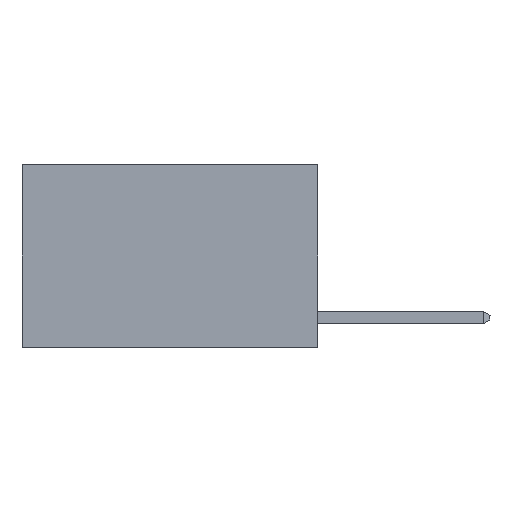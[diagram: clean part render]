
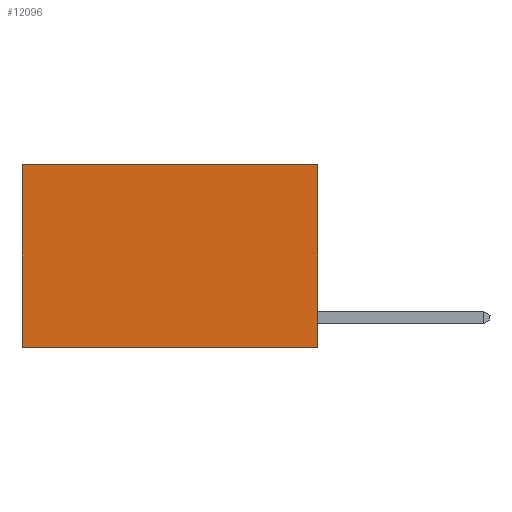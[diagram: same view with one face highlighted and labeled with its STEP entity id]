
A CAD part, left-side view. The second image highlights one B-rep face of the part: STEP entity #12096.
In plain terms, the highlighted planar face has unit normal (-1, 0, 0).
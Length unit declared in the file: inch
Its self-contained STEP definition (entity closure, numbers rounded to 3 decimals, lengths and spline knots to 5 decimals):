
#21 = LINE ( 'NONE', #401, #19808 ) ;
#174 = FACE_OUTER_BOUND ( 'NONE', #12239, .T. ) ;
#401 = CARTESIAN_POINT ( 'NONE',  ( 0.2625, 0., 0. ) ) ;
#759 = CARTESIAN_POINT ( 'NONE',  ( 0.2625, 0.6, -0.37 ) ) ;
#1038 = CARTESIAN_POINT ( 'NONE',  ( 0.2625, 0., 0. ) ) ;
#1250 = ORIENTED_EDGE ( 'NONE', *, *, #7501, .T. ) ;
#1968 = VERTEX_POINT ( 'NONE', #759 ) ;
#2121 = CARTESIAN_POINT ( 'NONE',  ( 0.2625, 0., 0. ) ) ;
#2324 = VECTOR ( 'NONE', #8483, 39.37008 ) ;
#2770 = CARTESIAN_POINT ( 'NONE',  ( 0.2625, 0., -0.37 ) ) ;
#3202 = CARTESIAN_POINT ( 'NONE',  ( 0.2625, 0.6, 0. ) ) ;
#5156 = ORIENTED_EDGE ( 'NONE', *, *, #19092, .T. ) ;
#6600 = LINE ( 'NONE', #16501, #2324 ) ;
#7501 = EDGE_CURVE ( 'NONE', #9893, #1968, #6600, .T. ) ;
#8483 = DIRECTION ( 'NONE',  ( 0., 0., -1. ) ) ;
#9771 = CARTESIAN_POINT ( 'NONE',  ( 0.2625, 0., 0. ) ) ;
#9893 = VERTEX_POINT ( 'NONE', #3202 ) ;
#10176 = CARTESIAN_POINT ( 'NONE',  ( 0.2625, 0., -0.37 ) ) ;
#10863 = LINE ( 'NONE', #1038, #15350 ) ;
#11800 = VERTEX_POINT ( 'NONE', #2770 ) ;
#12096 = ADVANCED_FACE ( 'NONE', ( #174 ), #15845, .F. ) ;
#12120 = LINE ( 'NONE', #10176, #20460 ) ;
#12239 = EDGE_LOOP ( 'NONE', ( #1250, #15117, #14851, #5156 ) ) ;
#14851 = ORIENTED_EDGE ( 'NONE', *, *, #17315, .F. ) ;
#15117 = ORIENTED_EDGE ( 'NONE', *, *, #21129, .F. ) ;
#15350 = VECTOR ( 'NONE', #18247, 39.37008 ) ;
#15845 = PLANE ( 'NONE',  #18969 ) ;
#16501 = CARTESIAN_POINT ( 'NONE',  ( 0.2625, 0.6, 0. ) ) ;
#16948 = VERTEX_POINT ( 'NONE', #2121 ) ;
#17315 = EDGE_CURVE ( 'NONE', #16948, #11800, #21, .T. ) ;
#18247 = DIRECTION ( 'NONE',  ( 0., 1., 0. ) ) ;
#18314 = DIRECTION ( 'NONE',  ( 0., 1., 0. ) ) ;
#18969 = AXIS2_PLACEMENT_3D ( 'NONE', #9771, #19324, #21571 ) ;
#19092 = EDGE_CURVE ( 'NONE', #16948, #9893, #10863, .T. ) ;
#19324 = DIRECTION ( 'NONE',  ( 1., 0., 0. ) ) ;
#19808 = VECTOR ( 'NONE', #23738, 39.37008 ) ;
#20460 = VECTOR ( 'NONE', #18314, 39.37008 ) ;
#21129 = EDGE_CURVE ( 'NONE', #11800, #1968, #12120, .T. ) ;
#21571 = DIRECTION ( 'NONE',  ( 0., 0., -1. ) ) ;
#23738 = DIRECTION ( 'NONE',  ( 0., 0., -1. ) ) ;
